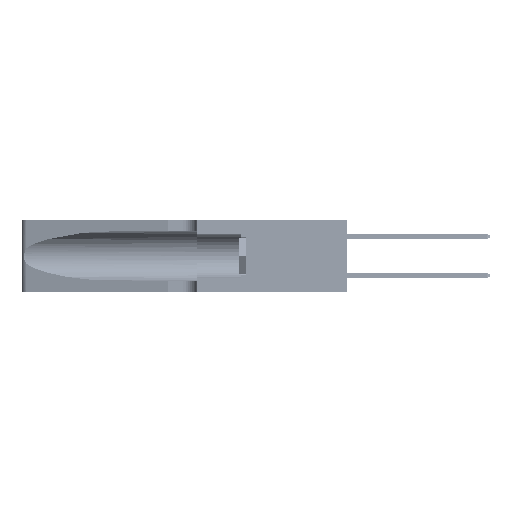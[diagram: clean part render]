
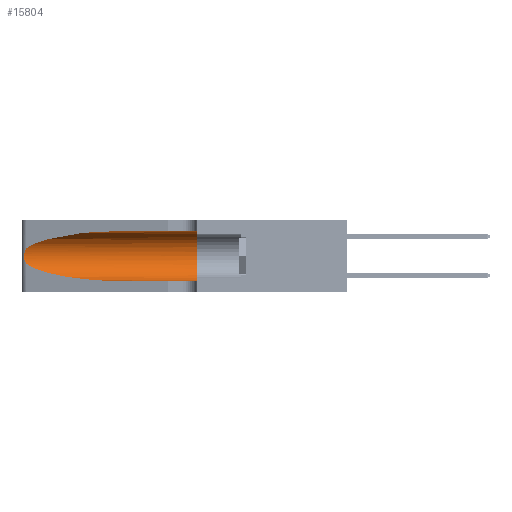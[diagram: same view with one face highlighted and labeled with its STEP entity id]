
A CAD part, left-side view. The second image highlights one B-rep face of the part: STEP entity #15804.
In plain terms, the highlighted cylindrical face has radius 3.308 mm (diameter 6.617 mm), a partial arc.
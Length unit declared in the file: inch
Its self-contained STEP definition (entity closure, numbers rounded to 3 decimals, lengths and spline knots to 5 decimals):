
#2496 = EDGE_CURVE ( 'NONE', #39733, #38882, #9499, .T. ) ;
#3518 = CARTESIAN_POINT ( 'NONE',  ( 0.26075, 1.23896, 0.178 ) ) ;
#4218 = CARTESIAN_POINT ( 'NONE',  ( 0.2373, 1.15595, 0.28018 ) ) ;
#5267 = DIRECTION ( 'NONE',  ( 0., -1., 0. ) ) ;
#5275 = AXIS2_PLACEMENT_3D ( 'NONE', #18741, #46788, #22790 ) ;
#6967 = EDGE_CURVE ( 'NONE', #14648, #27954, #47194, .T. ) ;
#7638 = CARTESIAN_POINT ( 'NONE',  ( 0.25856, 1.23593, 0.16098 ) ) ;
#9164 = CARTESIAN_POINT ( 'NONE',  ( 0.25487, 1.22718, 0.14631 ) ) ;
#9499 = LINE ( 'NONE', #14495, #39119 ) ;
#10283 = CARTESIAN_POINT ( 'NONE',  ( 0.1305, 1.61858, 0.31525 ) ) ;
#11717 = CARTESIAN_POINT ( 'NONE',  ( 0.25639, 1.23186, 0.15144 ) ) ;
#12359 = CARTESIAN_POINT ( 'NONE',  ( 0.1305, 0.72297, 0.31525 ) ) ;
#12713 = ORIENTED_EDGE ( 'NONE', *, *, #12896, .T. ) ;
#12896 = EDGE_CURVE ( 'NONE', #14648, #17392, #37727, .T. ) ;
#14495 = CARTESIAN_POINT ( 'NONE',  ( 0.1305, 1.61858, 0.05475 ) ) ;
#14648 = VERTEX_POINT ( 'NONE', #18315 ) ;
#15782 = CARTESIAN_POINT ( 'NONE',  ( 0.25487, 1.22718, 0.14631 ) ) ;
#15804 = ADVANCED_FACE ( 'NONE', ( #31121 ), #28613, .F. ) ;
#15866 = ORIENTED_EDGE ( 'NONE', *, *, #35987, .T. ) ;
#16119 = ORIENTED_EDGE ( 'NONE', *, *, #6967, .F. ) ;
#17334 = EDGE_CURVE ( 'NONE', #23415, #39733, #28407, .T. ) ;
#17392 = VERTEX_POINT ( 'NONE', #24685 ) ;
#18315 = CARTESIAN_POINT ( 'NONE',  ( 0.1305, 0.72297, 0.31525 ) ) ;
#18741 = CARTESIAN_POINT ( 'NONE',  ( 0.1305, 0.35, 0.185 ) ) ;
#19504 = CARTESIAN_POINT ( 'NONE',  ( 0.25555, 1.22994, 0.2215 ) ) ;
#19539 = CARTESIAN_POINT ( 'NONE',  ( 0.1305, 0.35, 0.31525 ) ) ;
#19672 = CARTESIAN_POINT ( 'NONE',  ( 0.25639, 1.23184, 0.21858 ) ) ;
#20334 = AXIS2_PLACEMENT_3D ( 'NONE', #33488, #5267, #49367 ) ;
#21930 = EDGE_LOOP ( 'NONE', ( #12713, #15866, #33405, #28622, #34949, #16119 ) ) ;
#22438 = DIRECTION ( 'NONE',  ( 0., -1., 0. ) ) ;
#22645 = CARTESIAN_POINT ( 'NONE',  ( 0.25487, 1.22718, 0.14631 ) ) ;
#22790 = DIRECTION ( 'NONE',  ( 0., 0., 1. ) ) ;
#23415 = VERTEX_POINT ( 'NONE', #22645 ) ;
#23713 = CARTESIAN_POINT ( 'NONE',  ( 0.25854, 1.2359, 0.20912 ) ) ;
#24330 = CARTESIAN_POINT ( 'NONE',  ( 0.2373, 1.15595, 0.08982 ) ) ;
#24492 = B_SPLINE_CURVE_WITH_KNOTS ( 'NONE', 3,
 ( #35678, #19504, #19672, #47713, #23713, #51704, #27822, #3518, #31815, #7638, #35846, #11717, #39880, #15782 ),
 .UNSPECIFIED., .F., .F.,
 ( 4, 2, 2, 2, 2, 2, 4 ),
 ( 0., 0.00027, 0.00053, 0.00107, 0.0016, 0.00187, 0.00214 ),
 .UNSPECIFIED. ) ;
#24685 = CARTESIAN_POINT ( 'NONE',  ( 0.25487, 1.22718, 0.22369 ) ) ;
#26211 = CARTESIAN_POINT ( 'NONE',  ( 0.1305, 0.72297, 0.05475 ) ) ;
#27822 = CARTESIAN_POINT ( 'NONE',  ( 0.26075, 1.23896, 0.19203 ) ) ;
#27954 = VERTEX_POINT ( 'NONE', #19539 ) ;
#28407 =( BOUNDED_CURVE ( )  B_SPLINE_CURVE ( 3, ( #9164, #24330, #32250, #28412 ),
 .UNSPECIFIED., .F., .T. ) 
 B_SPLINE_CURVE_WITH_KNOTS ( ( 4, 4 ),
 ( 3.44316, 4.71239 ),
 .UNSPECIFIED. ) 
 CURVE ( )  GEOMETRIC_REPRESENTATION_ITEM ( )  RATIONAL_B_SPLINE_CURVE ( ( 1., 0.87, 0.87, 1. ) ) 
 REPRESENTATION_ITEM ( '' )  );
#28412 = CARTESIAN_POINT ( 'NONE',  ( 0.1305, 0.72297, 0.05475 ) ) ;
#28613 = CYLINDRICAL_SURFACE ( 'NONE', #20334, 0.13025 ) ;
#28622 = ORIENTED_EDGE ( 'NONE', *, *, #2496, .T. ) ;
#31121 = FACE_OUTER_BOUND ( 'NONE', #21930, .T. ) ;
#31815 = CARTESIAN_POINT ( 'NONE',  ( 0.26017, 1.23833, 0.17102 ) ) ;
#32250 = CARTESIAN_POINT ( 'NONE',  ( 0.18966, 0.96281, 0.05475 ) ) ;
#33405 = ORIENTED_EDGE ( 'NONE', *, *, #17334, .T. ) ;
#33488 = CARTESIAN_POINT ( 'NONE',  ( 0.1305, 1.61858, 0.185 ) ) ;
#34949 = ORIENTED_EDGE ( 'NONE', *, *, #45547, .F. ) ;
#35678 = CARTESIAN_POINT ( 'NONE',  ( 0.25487, 1.22718, 0.22369 ) ) ;
#35846 = CARTESIAN_POINT ( 'NONE',  ( 0.25789, 1.23486, 0.15765 ) ) ;
#35987 = EDGE_CURVE ( 'NONE', #17392, #23415, #24492, .T. ) ;
#36493 = CARTESIAN_POINT ( 'NONE',  ( 0.18966, 0.96281, 0.31525 ) ) ;
#36576 = VECTOR ( 'NONE', #46462, 39.37008 ) ;
#37727 =( BOUNDED_CURVE ( )  B_SPLINE_CURVE ( 3, ( #12359, #36493, #4218, #40540 ),
 .UNSPECIFIED., .F., .F. ) 
 B_SPLINE_CURVE_WITH_KNOTS ( ( 4, 4 ),
 ( 1.5708, 2.84003 ),
 .UNSPECIFIED. ) 
 CURVE ( )  GEOMETRIC_REPRESENTATION_ITEM ( )  RATIONAL_B_SPLINE_CURVE ( ( 1., 0.87, 0.87, 1. ) ) 
 REPRESENTATION_ITEM ( '' )  );
#38882 = VERTEX_POINT ( 'NONE', #40995 ) ;
#39119 = VECTOR ( 'NONE', #22438, 39.37008 ) ;
#39733 = VERTEX_POINT ( 'NONE', #26211 ) ;
#39880 = CARTESIAN_POINT ( 'NONE',  ( 0.25555, 1.22993, 0.14849 ) ) ;
#40540 = CARTESIAN_POINT ( 'NONE',  ( 0.25487, 1.22718, 0.22369 ) ) ;
#40945 = CIRCLE ( 'NONE', #5275, 0.13025 ) ;
#40995 = CARTESIAN_POINT ( 'NONE',  ( 0.1305, 0.35, 0.05475 ) ) ;
#45547 = EDGE_CURVE ( 'NONE', #27954, #38882, #40945, .T. ) ;
#46462 = DIRECTION ( 'NONE',  ( 0., -1., 0. ) ) ;
#46788 = DIRECTION ( 'NONE',  ( 0., 1., 0. ) ) ;
#47194 = LINE ( 'NONE', #10283, #36576 ) ;
#47713 = CARTESIAN_POINT ( 'NONE',  ( 0.25787, 1.23484, 0.2124 ) ) ;
#49367 = DIRECTION ( 'NONE',  ( 0., 0., -1. ) ) ;
#51704 = CARTESIAN_POINT ( 'NONE',  ( 0.26018, 1.23835, 0.19895 ) ) ;
